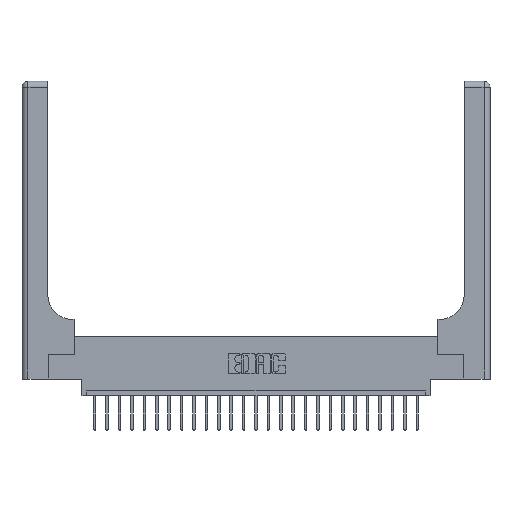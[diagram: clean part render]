
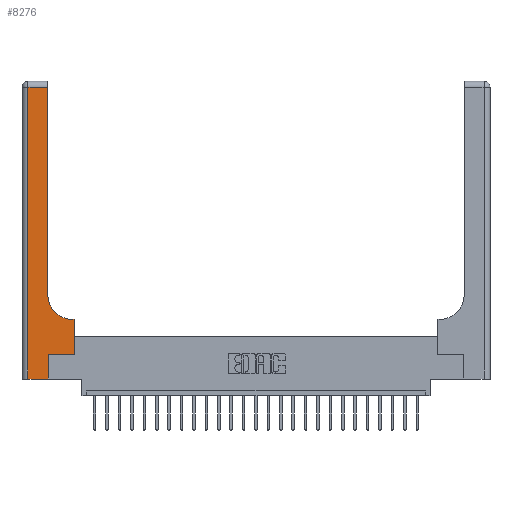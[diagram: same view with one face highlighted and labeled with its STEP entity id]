
A CAD part, top view. The second image highlights one B-rep face of the part: STEP entity #8276.
In plain terms, the highlighted planar face has unit normal (0, 0, 1).
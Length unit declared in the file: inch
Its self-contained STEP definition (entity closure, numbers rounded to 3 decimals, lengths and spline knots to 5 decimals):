
#89 = AXIS2_PLACEMENT_3D ( 'NONE', #2981, #19987, #18192 ) ;
#201 = DIRECTION ( 'NONE',  ( -1., 0., 0. ) ) ;
#382 = CARTESIAN_POINT ( 'NONE',  ( 0.528, 0.25, 0.37 ) ) ;
#1146 = DIRECTION ( 'NONE',  ( 0., 1., 0. ) ) ;
#1149 = DIRECTION ( 'NONE',  ( 0., 1., 0. ) ) ;
#1722 = LINE ( 'NONE', #16585, #6132 ) ;
#1765 = CARTESIAN_POINT ( 'NONE',  ( 0.06, 3., 0.37 ) ) ;
#2117 = DIRECTION ( 'NONE',  ( 1., 0., 0. ) ) ;
#2300 = CARTESIAN_POINT ( 'NONE',  ( 0.26, 2.94, 0.37 ) ) ;
#2835 = VECTOR ( 'NONE', #1146, 39.37008 ) ;
#2981 = CARTESIAN_POINT ( 'NONE',  ( 0.51, 0.85, 0.37 ) ) ;
#3093 = LINE ( 'NONE', #20909, #16772 ) ;
#3272 = CARTESIAN_POINT ( 'NONE',  ( 0.265, 0., 0.37 ) ) ;
#3394 = FACE_OUTER_BOUND ( 'NONE', #5627, .T. ) ;
#3646 = VERTEX_POINT ( 'NONE', #22928 ) ;
#4359 = LINE ( 'NONE', #13283, #21493 ) ;
#4371 = CARTESIAN_POINT ( 'NONE',  ( 0.528, 0.25, 0.37 ) ) ;
#4819 = AXIS2_PLACEMENT_3D ( 'NONE', #10154, #23144, #15864 ) ;
#5050 = VERTEX_POINT ( 'NONE', #16035 ) ;
#5162 = LINE ( 'NONE', #382, #11264 ) ;
#5223 = CARTESIAN_POINT ( 'NONE',  ( 0.26, 3., 0.37 ) ) ;
#5338 = EDGE_CURVE ( 'NONE', #3646, #15860, #21798, .T. ) ;
#5627 = EDGE_LOOP ( 'NONE', ( #14390, #10200, #14197, #8850, #19715, #19989, #21418, #13238, #21311 ) ) ;
#5736 = CARTESIAN_POINT ( 'NONE',  ( 0.265, 0.25, 0.37 ) ) ;
#5762 = EDGE_CURVE ( 'NONE', #5050, #3646, #4359, .T. ) ;
#5783 = CARTESIAN_POINT ( 'NONE',  ( 0.51, 0.6, 0.37 ) ) ;
#6132 = VECTOR ( 'NONE', #201, 39.37008 ) ;
#6353 = LINE ( 'NONE', #5223, #2835 ) ;
#6713 = VECTOR ( 'NONE', #1149, 39.37008 ) ;
#7403 = VERTEX_POINT ( 'NONE', #18860 ) ;
#8276 = ADVANCED_FACE ( 'NONE', ( #3394 ), #19591, .F. ) ;
#8324 = EDGE_CURVE ( 'NONE', #9169, #7403, #18520, .T. ) ;
#8575 = VERTEX_POINT ( 'NONE', #2300 ) ;
#8850 = ORIENTED_EDGE ( 'NONE', *, *, #5762, .T. ) ;
#9169 = VERTEX_POINT ( 'NONE', #5783 ) ;
#9177 = CARTESIAN_POINT ( 'NONE',  ( 0.06, 2.94, 0.37 ) ) ;
#9311 = VERTEX_POINT ( 'NONE', #22319 ) ;
#9394 = EDGE_CURVE ( 'NONE', #8575, #12090, #17992, .T. ) ;
#9797 = DIRECTION ( 'NONE',  ( 1., 0., 0. ) ) ;
#10154 = CARTESIAN_POINT ( 'NONE',  ( 0., 3., 0.37 ) ) ;
#10179 = EDGE_CURVE ( 'NONE', #20662, #9311, #5162, .T. ) ;
#10200 = ORIENTED_EDGE ( 'NONE', *, *, #9394, .T. ) ;
#10820 = EDGE_CURVE ( 'NONE', #7403, #8575, #6353, .T. ) ;
#11107 = EDGE_CURVE ( 'NONE', #12090, #5050, #11536, .T. ) ;
#11264 = VECTOR ( 'NONE', #17255, 39.37008 ) ;
#11298 = DIRECTION ( 'NONE',  ( 0., -1., 0. ) ) ;
#11536 = LINE ( 'NONE', #1765, #21405 ) ;
#12090 = VERTEX_POINT ( 'NONE', #9177 ) ;
#13238 = ORIENTED_EDGE ( 'NONE', *, *, #19097, .T. ) ;
#13283 = CARTESIAN_POINT ( 'NONE',  ( 0., 0., 0.37 ) ) ;
#14197 = ORIENTED_EDGE ( 'NONE', *, *, #11107, .T. ) ;
#14390 = ORIENTED_EDGE ( 'NONE', *, *, #10820, .T. ) ;
#15860 = VERTEX_POINT ( 'NONE', #5736 ) ;
#15864 = DIRECTION ( 'NONE',  ( -1., 0., 0. ) ) ;
#16035 = CARTESIAN_POINT ( 'NONE',  ( 0.06, 0., 0.37 ) ) ;
#16585 = CARTESIAN_POINT ( 'NONE',  ( 0.26, 0.6, 0.37 ) ) ;
#16772 = VECTOR ( 'NONE', #9797, 39.37008 ) ;
#17255 = DIRECTION ( 'NONE',  ( 0., 1., 0. ) ) ;
#17992 = LINE ( 'NONE', #18234, #20902 ) ;
#18192 = DIRECTION ( 'NONE',  ( 1., 0., 0. ) ) ;
#18234 = CARTESIAN_POINT ( 'NONE',  ( 0., 2.94, 0.37 ) ) ;
#18520 = CIRCLE ( 'NONE', #89, 0.25 ) ;
#18860 = CARTESIAN_POINT ( 'NONE',  ( 0.26, 0.85, 0.37 ) ) ;
#19097 = EDGE_CURVE ( 'NONE', #9311, #9169, #1722, .T. ) ;
#19591 = PLANE ( 'NONE',  #4819 ) ;
#19715 = ORIENTED_EDGE ( 'NONE', *, *, #5338, .T. ) ;
#19987 = DIRECTION ( 'NONE',  ( 0., 0., -1. ) ) ;
#19989 = ORIENTED_EDGE ( 'NONE', *, *, #21286, .T. ) ;
#20123 = DIRECTION ( 'NONE',  ( -1., 0., 0. ) ) ;
#20662 = VERTEX_POINT ( 'NONE', #4371 ) ;
#20902 = VECTOR ( 'NONE', #20123, 39.37008 ) ;
#20909 = CARTESIAN_POINT ( 'NONE',  ( 0.265, 0.25, 0.37 ) ) ;
#21286 = EDGE_CURVE ( 'NONE', #15860, #20662, #3093, .T. ) ;
#21311 = ORIENTED_EDGE ( 'NONE', *, *, #8324, .T. ) ;
#21405 = VECTOR ( 'NONE', #11298, 39.37008 ) ;
#21418 = ORIENTED_EDGE ( 'NONE', *, *, #10179, .T. ) ;
#21493 = VECTOR ( 'NONE', #2117, 39.37008 ) ;
#21798 = LINE ( 'NONE', #3272, #6713 ) ;
#22319 = CARTESIAN_POINT ( 'NONE',  ( 0.528, 0.6, 0.37 ) ) ;
#22928 = CARTESIAN_POINT ( 'NONE',  ( 0.265, 0., 0.37 ) ) ;
#23144 = DIRECTION ( 'NONE',  ( 0., 0., -1. ) ) ;
